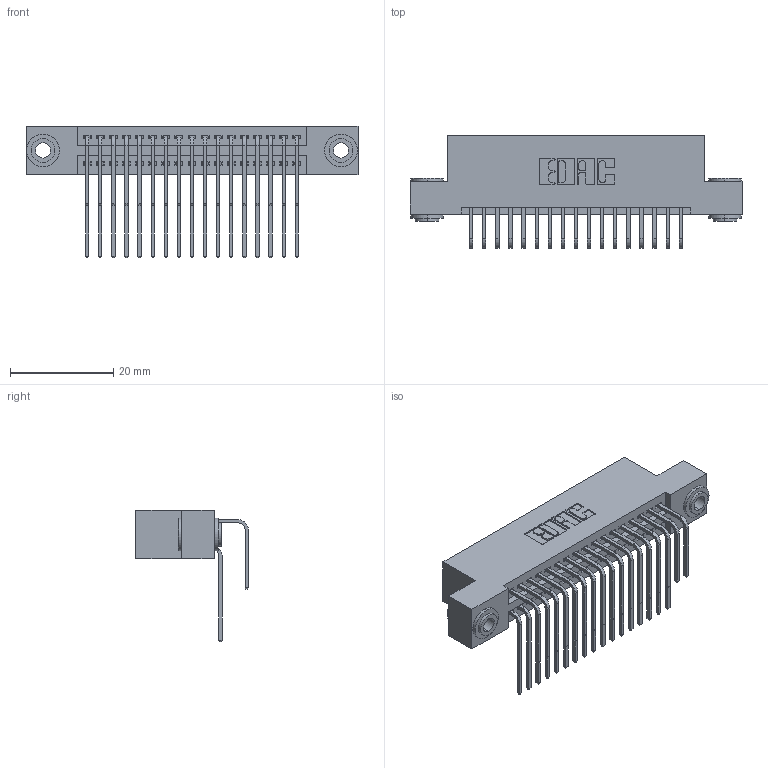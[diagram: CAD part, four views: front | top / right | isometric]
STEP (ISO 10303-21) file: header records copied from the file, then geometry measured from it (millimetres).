
FILE_DESCRIPTION (( 'STEP AP203' ), '1' );
FILE_NAME ('345-034-558-203.STEP', '2019-10-28T10:37:33', ( '' ), ( '' ), 'SwSTEP 2.0', 'SolidWorks 2016', '' );
FILE_SCHEMA (( 'CONFIG_CONTROL_DESIGN' ));
Length unit declared in the file: inch
Products named in the file (5): 345-292-001_558 559 Tail - 1; 345 Part_Flush Mounting Lugs - 0.156 Dia-TH; 345-250-002_345-250-002-102; 345-292-001_558 Tail - 2; 345-034-558-203
Assembly tree (37 placements, depth 2):
  345-034-558-203
    345 Part_Flush Mounting Lugs - 0.156 Dia-TH
    345-292-001_558 559 Tail - 1  x17
    345-292-001_558 Tail - 2  x17
    345-250-002_345-250-002-102  x2
Bounding box: 64.39 x 21.83 x 25.53 mm (x, y, z)
Volume: 6238.3 mm3; surface area: 9864.2 mm2
Topology: 37 solids, 37 shells, 1932 faces, 5687 edges, 3742 vertices
Faces by surface type: plane 1280, cylinder 644, cone 8
Entity records: 19006 total; most frequent: CARTESIAN_POINT 3230, ORIENTED_EDGE 3106, DIRECTION 2883, EDGE_CURVE 1553, LINE 1289, VECTOR 1289, VERTEX_POINT 1030, AXIS2_PLACEMENT_3D 797
